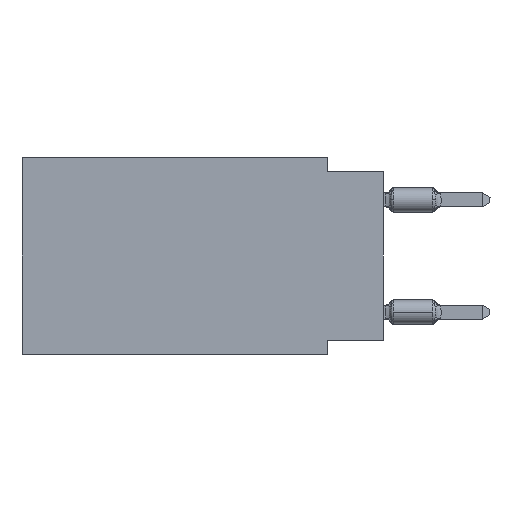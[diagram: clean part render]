
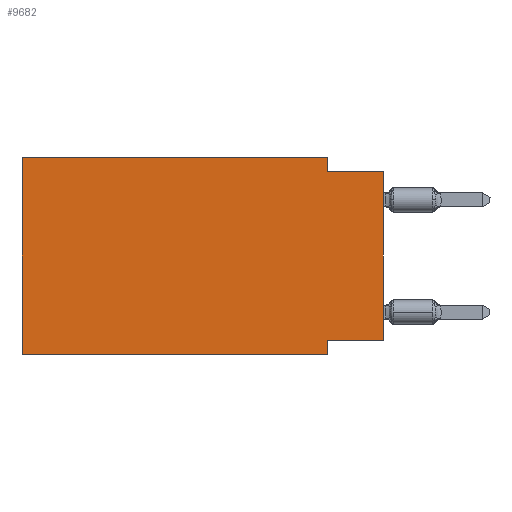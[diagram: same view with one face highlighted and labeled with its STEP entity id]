
A CAD part, left-side view. The second image highlights one B-rep face of the part: STEP entity #9682.
In plain terms, the highlighted planar face has unit normal (-1, 0, 0).
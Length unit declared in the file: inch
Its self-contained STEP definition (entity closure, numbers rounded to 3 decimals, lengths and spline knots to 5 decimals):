
#21 = AXIS2_PLACEMENT_3D ( 'NONE', #15979, #12232, #15851 ) ;
#131 = EDGE_CURVE ( 'NONE', #15683, #21099, #1020, .T. ) ;
#374 = VECTOR ( 'NONE', #10468, 39.37008 ) ;
#974 = LINE ( 'NONE', #13075, #18566 ) ;
#1004 = ORIENTED_EDGE ( 'NONE', *, *, #25315, .T. ) ;
#1020 = LINE ( 'NONE', #17674, #12702 ) ;
#1077 = CARTESIAN_POINT ( 'NONE',  ( 0., 0.1, -0.35 ) ) ;
#1088 = DIRECTION ( 'NONE',  ( 0., 1., 0. ) ) ;
#1664 = CARTESIAN_POINT ( 'NONE',  ( 0., 0., -0.325 ) ) ;
#1751 = ORIENTED_EDGE ( 'NONE', *, *, #9117, .F. ) ;
#2102 = VECTOR ( 'NONE', #8964, 39.37008 ) ;
#2734 = VECTOR ( 'NONE', #1088, 39.37008 ) ;
#3214 = EDGE_CURVE ( 'NONE', #12425, #15683, #6705, .T. ) ;
#3649 = CARTESIAN_POINT ( 'NONE',  ( 0., 0., -0.025 ) ) ;
#4038 = PLANE ( 'NONE',  #21 ) ;
#4143 = VERTEX_POINT ( 'NONE', #12049 ) ;
#4161 = EDGE_CURVE ( 'NONE', #23290, #19844, #20238, .T. ) ;
#4755 = VECTOR ( 'NONE', #5157, 39.37008 ) ;
#4994 = ORIENTED_EDGE ( 'NONE', *, *, #17920, .F. ) ;
#5062 = CARTESIAN_POINT ( 'NONE',  ( 0., 0.645, 0. ) ) ;
#5157 = DIRECTION ( 'NONE',  ( 0., 0., -1. ) ) ;
#5428 = ORIENTED_EDGE ( 'NONE', *, *, #4161, .F. ) ;
#5430 = CARTESIAN_POINT ( 'NONE',  ( 0., 0.1, 0. ) ) ;
#6028 = DIRECTION ( 'NONE',  ( 0., -1., 0. ) ) ;
#6705 = LINE ( 'NONE', #5062, #2102 ) ;
#6950 = EDGE_CURVE ( 'NONE', #11544, #4143, #13177, .T. ) ;
#8964 = DIRECTION ( 'NONE',  ( 0., 0., 1. ) ) ;
#9005 = ORIENTED_EDGE ( 'NONE', *, *, #3214, .F. ) ;
#9117 = EDGE_CURVE ( 'NONE', #21099, #23290, #13083, .T. ) ;
#9189 = DIRECTION ( 'NONE',  ( 0., -1., 0. ) ) ;
#9373 = CARTESIAN_POINT ( 'NONE',  ( 0., 0., 0. ) ) ;
#9682 = ADVANCED_FACE ( 'NONE', ( #17872 ), #4038, .F. ) ;
#10058 = ORIENTED_EDGE ( 'NONE', *, *, #10150, .T. ) ;
#10125 = ORIENTED_EDGE ( 'NONE', *, *, #131, .F. ) ;
#10150 = EDGE_CURVE ( 'NONE', #11544, #19844, #15528, .T. ) ;
#10468 = DIRECTION ( 'NONE',  ( 0., 0., -1. ) ) ;
#10725 = CARTESIAN_POINT ( 'NONE',  ( 0., 0.1, 0. ) ) ;
#11084 = CARTESIAN_POINT ( 'NONE',  ( 0., 0.1, -0.35 ) ) ;
#11544 = VERTEX_POINT ( 'NONE', #1664 ) ;
#12049 = CARTESIAN_POINT ( 'NONE',  ( 0., 0.1, -0.325 ) ) ;
#12068 = VECTOR ( 'NONE', #21429, 39.37008 ) ;
#12232 = DIRECTION ( 'NONE',  ( 1., 0., 0. ) ) ;
#12425 = VERTEX_POINT ( 'NONE', #17986 ) ;
#12593 = LINE ( 'NONE', #11084, #374 ) ;
#12702 = VECTOR ( 'NONE', #23589, 39.37008 ) ;
#13075 = CARTESIAN_POINT ( 'NONE',  ( 0., 0.645, -0.35 ) ) ;
#13083 = LINE ( 'NONE', #5430, #4755 ) ;
#13177 = LINE ( 'NONE', #23513, #2734 ) ;
#13533 = VERTEX_POINT ( 'NONE', #1077 ) ;
#13649 = CARTESIAN_POINT ( 'NONE',  ( 0., 0.1, -0.025 ) ) ;
#14074 = CARTESIAN_POINT ( 'NONE',  ( 0., 0., -0.025 ) ) ;
#15105 = ORIENTED_EDGE ( 'NONE', *, *, #6950, .F. ) ;
#15528 = LINE ( 'NONE', #9373, #12068 ) ;
#15683 = VERTEX_POINT ( 'NONE', #19328 ) ;
#15851 = DIRECTION ( 'NONE',  ( 0., 0., -1. ) ) ;
#15979 = CARTESIAN_POINT ( 'NONE',  ( 0., 0.645, 0. ) ) ;
#17079 = EDGE_LOOP ( 'NONE', ( #10058, #5428, #1751, #10125, #9005, #1004, #4994, #15105 ) ) ;
#17674 = CARTESIAN_POINT ( 'NONE',  ( 0., 0.645, 0. ) ) ;
#17872 = FACE_OUTER_BOUND ( 'NONE', #17079, .T. ) ;
#17920 = EDGE_CURVE ( 'NONE', #4143, #13533, #12593, .T. ) ;
#17986 = CARTESIAN_POINT ( 'NONE',  ( 0., 0.645, -0.35 ) ) ;
#18566 = VECTOR ( 'NONE', #9189, 39.37008 ) ;
#19328 = CARTESIAN_POINT ( 'NONE',  ( 0., 0.645, 0. ) ) ;
#19844 = VERTEX_POINT ( 'NONE', #3649 ) ;
#20238 = LINE ( 'NONE', #14074, #25641 ) ;
#21099 = VERTEX_POINT ( 'NONE', #10725 ) ;
#21429 = DIRECTION ( 'NONE',  ( 0., 0., 1. ) ) ;
#23290 = VERTEX_POINT ( 'NONE', #13649 ) ;
#23513 = CARTESIAN_POINT ( 'NONE',  ( 0., 0., -0.325 ) ) ;
#23589 = DIRECTION ( 'NONE',  ( 0., -1., 0. ) ) ;
#25315 = EDGE_CURVE ( 'NONE', #12425, #13533, #974, .T. ) ;
#25641 = VECTOR ( 'NONE', #6028, 39.37008 ) ;
